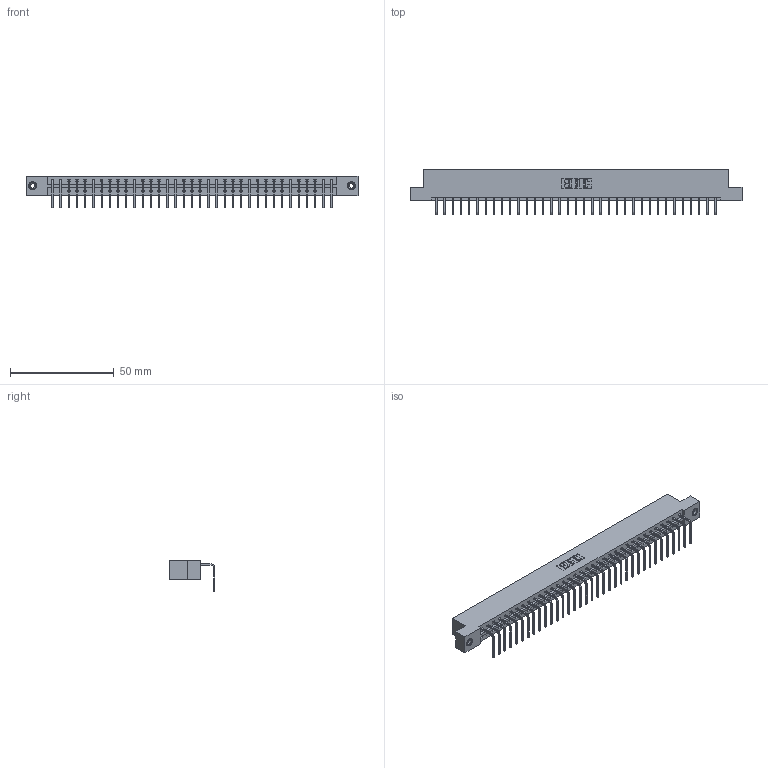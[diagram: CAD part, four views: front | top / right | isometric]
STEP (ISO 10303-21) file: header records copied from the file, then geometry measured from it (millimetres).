
FILE_DESCRIPTION (( 'STEP AP203' ), '1' );
FILE_NAME ('833-035-558-108.STEP', '2020-06-03T01:06:32', ( '' ), ( '' ), 'SwSTEP 2.0', 'SolidWorks 2020', '' );
FILE_SCHEMA (( 'CONFIG_CONTROL_DESIGN' ));
Length unit declared in the file: inch
Products named in the file (4): 833 Part_Flush - .156 Dia - TI; 345-292-001_558 Tail - 2; 345-250-001_345-250-003-102; 833-035-558-108
Assembly tree (38 placements, depth 2):
  833-035-558-108
    833 Part_Flush - .156 Dia - TI
    345-292-001_558 Tail - 2  x35
    345-250-001_345-250-003-102  x2
Bounding box: 160.22 x 22.17 x 15.37 mm (x, y, z)
Volume: 16172.9 mm3; surface area: 18193.9 mm2
Topology: 38 solids, 38 shells, 2274 faces, 6817 edges, 4490 vertices
Faces by surface type: plane 1642, cylinder 616, cone 12, torus 4
Entity records: 23572 total; most frequent: CARTESIAN_POINT 4050, ORIENTED_EDGE 4014, DIRECTION 3463, EDGE_CURVE 2007, LINE 1859, VECTOR 1859, VERTEX_POINT 1332, AXIS2_PLACEMENT_3D 802
